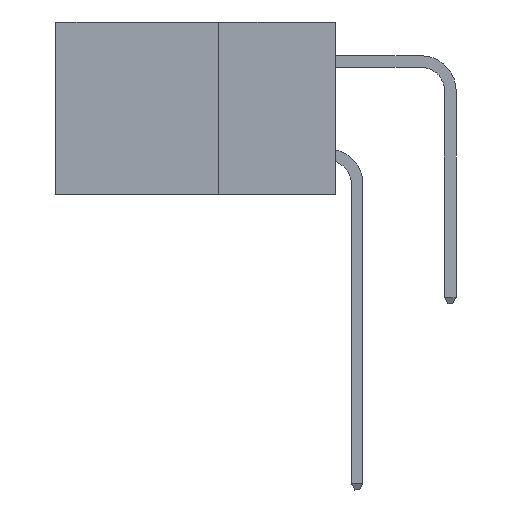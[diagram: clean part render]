
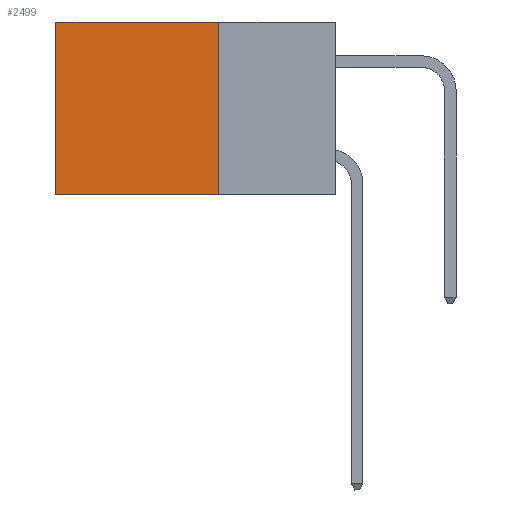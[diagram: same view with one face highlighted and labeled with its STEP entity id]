
A CAD part, left-side view. The second image highlights one B-rep face of the part: STEP entity #2499.
In plain terms, the highlighted planar face has unit normal (-1, 0, 0).
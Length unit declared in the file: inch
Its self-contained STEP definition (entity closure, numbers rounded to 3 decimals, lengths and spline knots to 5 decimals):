
#1053 = VERTEX_POINT ( 'NONE', #7306 ) ;
#2244 = CARTESIAN_POINT ( 'NONE',  ( 0.2875, 0.6, -0.37 ) ) ;
#2499 = ADVANCED_FACE ( 'NONE', ( #5564 ), #14621, .F. ) ;
#2552 = CARTESIAN_POINT ( 'NONE',  ( 0.2875, 0.6, 0. ) ) ;
#2644 = LINE ( 'NONE', #2552, #11096 ) ;
#3540 = DIRECTION ( 'NONE',  ( 0., 1., 0. ) ) ;
#5564 = FACE_OUTER_BOUND ( 'NONE', #12810, .T. ) ;
#5718 = ORIENTED_EDGE ( 'NONE', *, *, #23414, .T. ) ;
#5920 = DIRECTION ( 'NONE',  ( 0., 0., -1. ) ) ;
#7306 = CARTESIAN_POINT ( 'NONE',  ( 0.2875, 0.25, -0.37 ) ) ;
#7474 = VERTEX_POINT ( 'NONE', #10297 ) ;
#9237 = DIRECTION ( 'NONE',  ( 0., 0., -1. ) ) ;
#9279 = EDGE_CURVE ( 'NONE', #1053, #11290, #15899, .T. ) ;
#10261 = AXIS2_PLACEMENT_3D ( 'NONE', #19242, #22890, #9237 ) ;
#10297 = CARTESIAN_POINT ( 'NONE',  ( 0.2875, 0.25, 0. ) ) ;
#11096 = VECTOR ( 'NONE', #13389, 39.37008 ) ;
#11284 = CARTESIAN_POINT ( 'NONE',  ( 0.2875, 0.25, 0. ) ) ;
#11290 = VERTEX_POINT ( 'NONE', #2244 ) ;
#12424 = ORIENTED_EDGE ( 'NONE', *, *, #9279, .F. ) ;
#12736 = CARTESIAN_POINT ( 'NONE',  ( 0.2875, 0.6, 0. ) ) ;
#12810 = EDGE_LOOP ( 'NONE', ( #5718, #12424, #18201, #15597 ) ) ;
#13303 = CARTESIAN_POINT ( 'NONE',  ( 0.2875, 0.25, 0. ) ) ;
#13389 = DIRECTION ( 'NONE',  ( 0., 0., -1. ) ) ;
#14621 = PLANE ( 'NONE',  #10261 ) ;
#15109 = DIRECTION ( 'NONE',  ( 0., 1., 0. ) ) ;
#15597 = ORIENTED_EDGE ( 'NONE', *, *, #17273, .T. ) ;
#15899 = LINE ( 'NONE', #23441, #20870 ) ;
#17273 = EDGE_CURVE ( 'NONE', #7474, #20077, #21702, .T. ) ;
#18201 = ORIENTED_EDGE ( 'NONE', *, *, #23305, .F. ) ;
#19242 = CARTESIAN_POINT ( 'NONE',  ( 0.2875, 0.25, 0. ) ) ;
#20077 = VERTEX_POINT ( 'NONE', #12736 ) ;
#20870 = VECTOR ( 'NONE', #3540, 39.37008 ) ;
#21130 = VECTOR ( 'NONE', #15109, 39.37008 ) ;
#21702 = LINE ( 'NONE', #13303, #21130 ) ;
#22535 = VECTOR ( 'NONE', #5920, 39.37008 ) ;
#22890 = DIRECTION ( 'NONE',  ( 1., 0., 0. ) ) ;
#23095 = LINE ( 'NONE', #11284, #22535 ) ;
#23305 = EDGE_CURVE ( 'NONE', #7474, #1053, #23095, .T. ) ;
#23414 = EDGE_CURVE ( 'NONE', #20077, #11290, #2644, .T. ) ;
#23441 = CARTESIAN_POINT ( 'NONE',  ( 0.2875, 0.25, -0.37 ) ) ;
